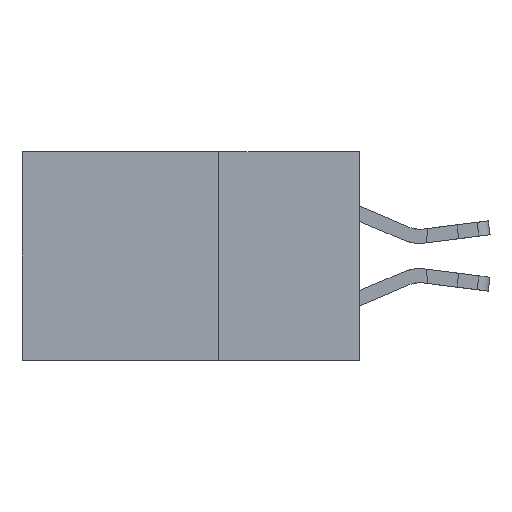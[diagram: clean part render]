
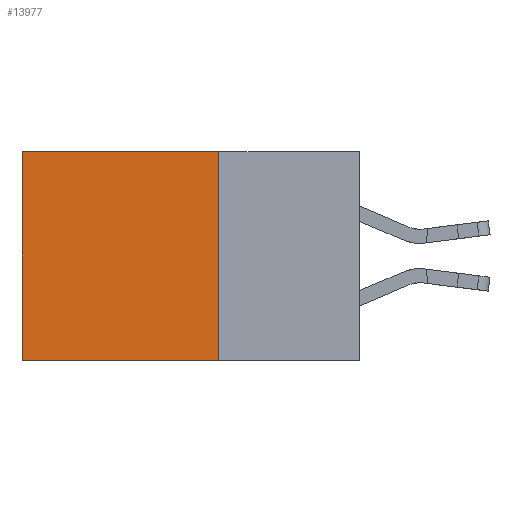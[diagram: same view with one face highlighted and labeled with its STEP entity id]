
A CAD part, left-side view. The second image highlights one B-rep face of the part: STEP entity #13977.
In plain terms, the highlighted planar face has unit normal (-1, 0, 0).
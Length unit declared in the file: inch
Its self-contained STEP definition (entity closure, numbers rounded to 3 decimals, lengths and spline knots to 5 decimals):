
#22 = CARTESIAN_POINT ( 'NONE',  ( 0.2875, 0.6, -0.37 ) ) ;
#245 = LINE ( 'NONE', #16621, #22433 ) ;
#1103 = EDGE_CURVE ( 'NONE', #6564, #6781, #16053, .T. ) ;
#1507 = FACE_OUTER_BOUND ( 'NONE', #20951, .T. ) ;
#1887 = VECTOR ( 'NONE', #16991, 39.37008 ) ;
#3145 = VECTOR ( 'NONE', #3986, 39.37008 ) ;
#3313 = ORIENTED_EDGE ( 'NONE', *, *, #1103, .F. ) ;
#3454 = VERTEX_POINT ( 'NONE', #17860 ) ;
#3582 = VECTOR ( 'NONE', #12104, 39.37008 ) ;
#3986 = DIRECTION ( 'NONE',  ( 0., 0., -1. ) ) ;
#6463 = VERTEX_POINT ( 'NONE', #12428 ) ;
#6564 = VERTEX_POINT ( 'NONE', #11287 ) ;
#6781 = VERTEX_POINT ( 'NONE', #22 ) ;
#7199 = CARTESIAN_POINT ( 'NONE',  ( 0.2875, 0.25, 0. ) ) ;
#9138 = DIRECTION ( 'NONE',  ( 0., 0., -1. ) ) ;
#10431 = ORIENTED_EDGE ( 'NONE', *, *, #14301, .T. ) ;
#10513 = ORIENTED_EDGE ( 'NONE', *, *, #17989, .T. ) ;
#10883 = LINE ( 'NONE', #14634, #3145 ) ;
#11287 = CARTESIAN_POINT ( 'NONE',  ( 0.2875, 0.25, -0.37 ) ) ;
#11304 = LINE ( 'NONE', #15147, #1887 ) ;
#11345 = DIRECTION ( 'NONE',  ( 0., 0., -1. ) ) ;
#12104 = DIRECTION ( 'NONE',  ( 0., 1., 0. ) ) ;
#12428 = CARTESIAN_POINT ( 'NONE',  ( 0.2875, 0.25, 0. ) ) ;
#12542 = DIRECTION ( 'NONE',  ( 1., 0., 0. ) ) ;
#13977 = ADVANCED_FACE ( 'NONE', ( #1507 ), #21524, .F. ) ;
#14301 = EDGE_CURVE ( 'NONE', #3454, #6781, #10883, .T. ) ;
#14634 = CARTESIAN_POINT ( 'NONE',  ( 0.2875, 0.6, 0. ) ) ;
#15147 = CARTESIAN_POINT ( 'NONE',  ( 0.2875, 0.25, 0. ) ) ;
#16053 = LINE ( 'NONE', #17277, #3582 ) ;
#16621 = CARTESIAN_POINT ( 'NONE',  ( 0.2875, 0.25, 0. ) ) ;
#16991 = DIRECTION ( 'NONE',  ( 0., 1., 0. ) ) ;
#17277 = CARTESIAN_POINT ( 'NONE',  ( 0.2875, 0.25, -0.37 ) ) ;
#17860 = CARTESIAN_POINT ( 'NONE',  ( 0.2875, 0.6, 0. ) ) ;
#17989 = EDGE_CURVE ( 'NONE', #6463, #3454, #11304, .T. ) ;
#20436 = ORIENTED_EDGE ( 'NONE', *, *, #21977, .F. ) ;
#20809 = AXIS2_PLACEMENT_3D ( 'NONE', #7199, #12542, #9138 ) ;
#20951 = EDGE_LOOP ( 'NONE', ( #10431, #3313, #20436, #10513 ) ) ;
#21524 = PLANE ( 'NONE',  #20809 ) ;
#21977 = EDGE_CURVE ( 'NONE', #6463, #6564, #245, .T. ) ;
#22433 = VECTOR ( 'NONE', #11345, 39.37008 ) ;
